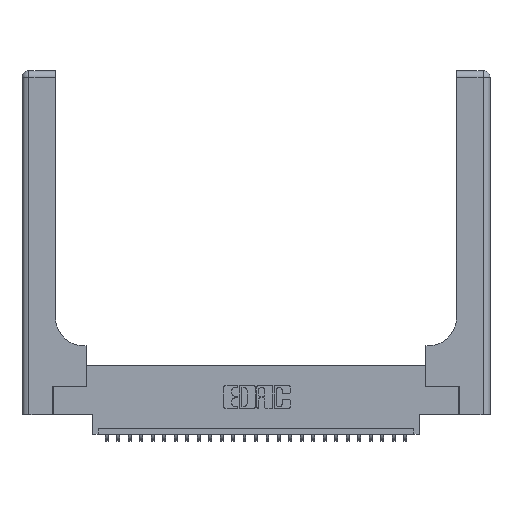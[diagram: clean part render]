
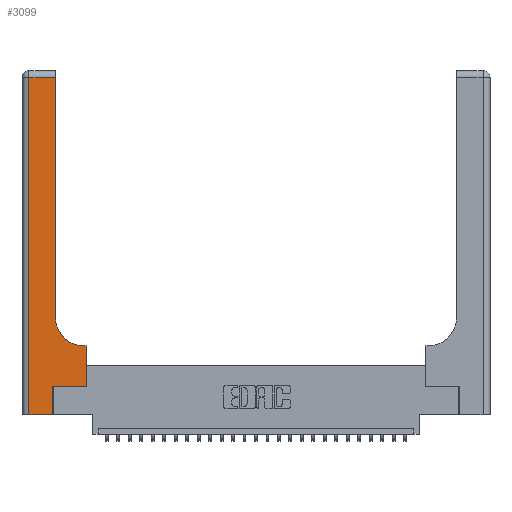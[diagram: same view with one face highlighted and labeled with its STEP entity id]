
A CAD part, top view. The second image highlights one B-rep face of the part: STEP entity #3099.
In plain terms, the highlighted planar face has unit normal (0, 0, 1).
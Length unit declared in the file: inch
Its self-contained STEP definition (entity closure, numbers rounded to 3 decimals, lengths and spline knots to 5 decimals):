
#48 = ORIENTED_EDGE ( 'NONE', *, *, #20366, .T. ) ;
#211 = CARTESIAN_POINT ( 'NONE',  ( 0.2915, 0.85, 0.37 ) ) ;
#516 = CARTESIAN_POINT ( 'NONE',  ( 0.5415, 0.85, 0.37 ) ) ;
#715 = DIRECTION ( 'NONE',  ( 0., 0., -1. ) ) ;
#718 = DIRECTION ( 'NONE',  ( 0., 0., -1. ) ) ;
#1083 = CARTESIAN_POINT ( 'NONE',  ( 0.06, 3., 0.37 ) ) ;
#1150 = EDGE_CURVE ( 'NONE', #22316, #1816, #16706, .T. ) ;
#1428 = FACE_OUTER_BOUND ( 'NONE', #13423, .T. ) ;
#1612 = DIRECTION ( 'NONE',  ( -1., 0., 0. ) ) ;
#1733 = ORIENTED_EDGE ( 'NONE', *, *, #14765, .T. ) ;
#1816 = VERTEX_POINT ( 'NONE', #25189 ) ;
#1866 = CARTESIAN_POINT ( 'NONE',  ( 0., 0., 0.37 ) ) ;
#2171 = CARTESIAN_POINT ( 'NONE',  ( 0.5585, 0.6, 0.37 ) ) ;
#2204 = EDGE_CURVE ( 'NONE', #24888, #22829, #15262, .T. ) ;
#2878 = CARTESIAN_POINT ( 'NONE',  ( 0.5415, 0.6, 0.37 ) ) ;
#3099 = ADVANCED_FACE ( 'NONE', ( #1428 ), #5391, .F. ) ;
#3220 = VECTOR ( 'NONE', #5137, 39.37008 ) ;
#3824 = VECTOR ( 'NONE', #5028, 39.37008 ) ;
#4271 = VECTOR ( 'NONE', #6434, 39.37008 ) ;
#4448 = ORIENTED_EDGE ( 'NONE', *, *, #1150, .T. ) ;
#5028 = DIRECTION ( 'NONE',  ( 0., 1., 0. ) ) ;
#5137 = DIRECTION ( 'NONE',  ( 0., 1., 0. ) ) ;
#5236 = VERTEX_POINT ( 'NONE', #211 ) ;
#5391 = PLANE ( 'NONE',  #15344 ) ;
#5777 = EDGE_CURVE ( 'NONE', #5236, #22316, #12655, .T. ) ;
#6114 = ORIENTED_EDGE ( 'NONE', *, *, #2204, .T. ) ;
#6403 = VERTEX_POINT ( 'NONE', #2171 ) ;
#6434 = DIRECTION ( 'NONE',  ( 1., 0., 0. ) ) ;
#6629 = DIRECTION ( 'NONE',  ( -1., 0., 0. ) ) ;
#7480 = ORIENTED_EDGE ( 'NONE', *, *, #12454, .T. ) ;
#7697 = ORIENTED_EDGE ( 'NONE', *, *, #18894, .T. ) ;
#9019 = CARTESIAN_POINT ( 'NONE',  ( 0.06, 0., 0.37 ) ) ;
#9250 = CARTESIAN_POINT ( 'NONE',  ( 0.5585, 0.25, 0.37 ) ) ;
#9319 = ORIENTED_EDGE ( 'NONE', *, *, #25384, .T. ) ;
#9422 = LINE ( 'NONE', #1083, #12429 ) ;
#12429 = VECTOR ( 'NONE', #22349, 39.37008 ) ;
#12454 = EDGE_CURVE ( 'NONE', #23737, #6403, #22967, .T. ) ;
#12589 = CIRCLE ( 'NONE', #16679, 0.25 ) ;
#12655 = LINE ( 'NONE', #18980, #13668 ) ;
#13393 = CARTESIAN_POINT ( 'NONE',  ( 0.269, 0., 0.37 ) ) ;
#13423 = EDGE_LOOP ( 'NONE', ( #20977, #4448, #1733, #9319, #6114, #24861, #7480, #48, #7697 ) ) ;
#13668 = VECTOR ( 'NONE', #21479, 39.37008 ) ;
#14168 = VECTOR ( 'NONE', #1612, 39.37008 ) ;
#14669 = DIRECTION ( 'NONE',  ( 1., 0., 0. ) ) ;
#14716 = CARTESIAN_POINT ( 'NONE',  ( 0.2915, 0.6, 0.37 ) ) ;
#14765 = EDGE_CURVE ( 'NONE', #1816, #21751, #9422, .T. ) ;
#15056 = CARTESIAN_POINT ( 'NONE',  ( 0., 2.94, 0.37 ) ) ;
#15262 = LINE ( 'NONE', #17641, #3220 ) ;
#15344 = AXIS2_PLACEMENT_3D ( 'NONE', #26475, #715, #20388 ) ;
#16679 = AXIS2_PLACEMENT_3D ( 'NONE', #516, #718, #24210 ) ;
#16706 = LINE ( 'NONE', #15056, #17384 ) ;
#17384 = VECTOR ( 'NONE', #6629, 39.37008 ) ;
#17450 = EDGE_CURVE ( 'NONE', #22829, #23737, #24015, .T. ) ;
#17641 = CARTESIAN_POINT ( 'NONE',  ( 0.269, 0., 0.37 ) ) ;
#18232 = LINE ( 'NONE', #14716, #14168 ) ;
#18704 = VECTOR ( 'NONE', #14669, 39.37008 ) ;
#18894 = EDGE_CURVE ( 'NONE', #18910, #5236, #12589, .T. ) ;
#18910 = VERTEX_POINT ( 'NONE', #2878 ) ;
#18980 = CARTESIAN_POINT ( 'NONE',  ( 0.2915, 3., 0.37 ) ) ;
#18986 = CARTESIAN_POINT ( 'NONE',  ( 0.269, 0.25, 0.37 ) ) ;
#19047 = CARTESIAN_POINT ( 'NONE',  ( 0.2915, 2.94, 0.37 ) ) ;
#20366 = EDGE_CURVE ( 'NONE', #6403, #18910, #18232, .T. ) ;
#20388 = DIRECTION ( 'NONE',  ( -1., 0., 0. ) ) ;
#20977 = ORIENTED_EDGE ( 'NONE', *, *, #5777, .T. ) ;
#21479 = DIRECTION ( 'NONE',  ( 0., 1., 0. ) ) ;
#21751 = VERTEX_POINT ( 'NONE', #9019 ) ;
#22316 = VERTEX_POINT ( 'NONE', #19047 ) ;
#22349 = DIRECTION ( 'NONE',  ( 0., -1., 0. ) ) ;
#22829 = VERTEX_POINT ( 'NONE', #25160 ) ;
#22967 = LINE ( 'NONE', #9250, #3824 ) ;
#23737 = VERTEX_POINT ( 'NONE', #25459 ) ;
#24015 = LINE ( 'NONE', #18986, #18704 ) ;
#24210 = DIRECTION ( 'NONE',  ( 1., 0., 0. ) ) ;
#24353 = LINE ( 'NONE', #1866, #4271 ) ;
#24861 = ORIENTED_EDGE ( 'NONE', *, *, #17450, .T. ) ;
#24888 = VERTEX_POINT ( 'NONE', #13393 ) ;
#25160 = CARTESIAN_POINT ( 'NONE',  ( 0.269, 0.25, 0.37 ) ) ;
#25189 = CARTESIAN_POINT ( 'NONE',  ( 0.06, 2.94, 0.37 ) ) ;
#25384 = EDGE_CURVE ( 'NONE', #21751, #24888, #24353, .T. ) ;
#25459 = CARTESIAN_POINT ( 'NONE',  ( 0.5585, 0.25, 0.37 ) ) ;
#26475 = CARTESIAN_POINT ( 'NONE',  ( 0., 3., 0.37 ) ) ;
